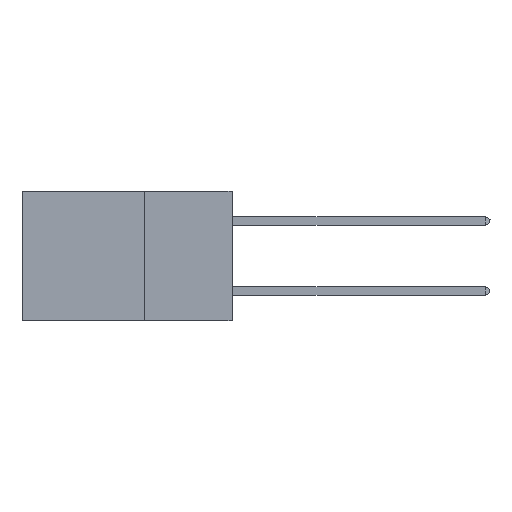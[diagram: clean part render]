
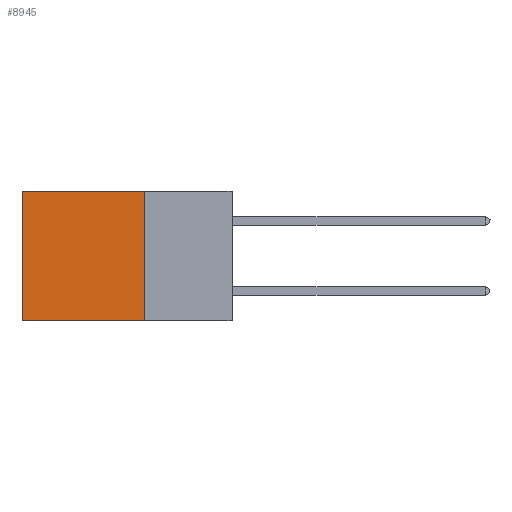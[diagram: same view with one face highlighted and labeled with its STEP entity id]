
A CAD part, left-side view. The second image highlights one B-rep face of the part: STEP entity #8945.
In plain terms, the highlighted planar face has unit normal (-1, 0, 0).
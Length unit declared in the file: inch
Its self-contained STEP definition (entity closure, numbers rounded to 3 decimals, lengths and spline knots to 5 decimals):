
#132 = EDGE_LOOP ( 'NONE', ( #12710, #3337, #16583, #10845 ) ) ;
#193 = EDGE_CURVE ( 'NONE', #6214, #15736, #16023, .T. ) ;
#449 = VECTOR ( 'NONE', #3916, 39.37008 ) ;
#1090 = EDGE_CURVE ( 'NONE', #14208, #12541, #8079, .T. ) ;
#1238 = CARTESIAN_POINT ( 'NONE',  ( 0.2875, 0.6, -0.37 ) ) ;
#1388 = AXIS2_PLACEMENT_3D ( 'NONE', #5143, #3465, #17423 ) ;
#1971 = EDGE_CURVE ( 'NONE', #12541, #15736, #16799, .T. ) ;
#3151 = DIRECTION ( 'NONE',  ( 0., 0., -1. ) ) ;
#3337 = ORIENTED_EDGE ( 'NONE', *, *, #193, .F. ) ;
#3465 = DIRECTION ( 'NONE',  ( 1., 0., 0. ) ) ;
#3916 = DIRECTION ( 'NONE',  ( 0., 0., -1. ) ) ;
#5143 = CARTESIAN_POINT ( 'NONE',  ( 0.2875, 0.25, 0. ) ) ;
#5452 = CARTESIAN_POINT ( 'NONE',  ( 0.2875, 0.25, -0.37 ) ) ;
#6214 = VERTEX_POINT ( 'NONE', #5452 ) ;
#6301 = CARTESIAN_POINT ( 'NONE',  ( 0.2875, 0.25, -0.37 ) ) ;
#7306 = CARTESIAN_POINT ( 'NONE',  ( 0.2875, 0.6, 0. ) ) ;
#8016 = VECTOR ( 'NONE', #8895, 39.37008 ) ;
#8079 = LINE ( 'NONE', #15164, #11753 ) ;
#8203 = VECTOR ( 'NONE', #3151, 39.37008 ) ;
#8895 = DIRECTION ( 'NONE',  ( 0., 1., 0. ) ) ;
#8945 = ADVANCED_FACE ( 'NONE', ( #12725 ), #15958, .F. ) ;
#9581 = DIRECTION ( 'NONE',  ( 0., 1., 0. ) ) ;
#10845 = ORIENTED_EDGE ( 'NONE', *, *, #1090, .T. ) ;
#11753 = VECTOR ( 'NONE', #9581, 39.37008 ) ;
#12430 = CARTESIAN_POINT ( 'NONE',  ( 0.2875, 0.6, 0. ) ) ;
#12432 = CARTESIAN_POINT ( 'NONE',  ( 0.2875, 0.25, 0. ) ) ;
#12541 = VERTEX_POINT ( 'NONE', #12430 ) ;
#12710 = ORIENTED_EDGE ( 'NONE', *, *, #1971, .T. ) ;
#12725 = FACE_OUTER_BOUND ( 'NONE', #132, .T. ) ;
#14073 = EDGE_CURVE ( 'NONE', #14208, #6214, #16596, .T. ) ;
#14208 = VERTEX_POINT ( 'NONE', #12432 ) ;
#15164 = CARTESIAN_POINT ( 'NONE',  ( 0.2875, 0.25, 0. ) ) ;
#15736 = VERTEX_POINT ( 'NONE', #1238 ) ;
#15958 = PLANE ( 'NONE',  #1388 ) ;
#16023 = LINE ( 'NONE', #6301, #8016 ) ;
#16583 = ORIENTED_EDGE ( 'NONE', *, *, #14073, .F. ) ;
#16596 = LINE ( 'NONE', #17733, #449 ) ;
#16799 = LINE ( 'NONE', #7306, #8203 ) ;
#17423 = DIRECTION ( 'NONE',  ( 0., 0., -1. ) ) ;
#17733 = CARTESIAN_POINT ( 'NONE',  ( 0.2875, 0.25, 0. ) ) ;
